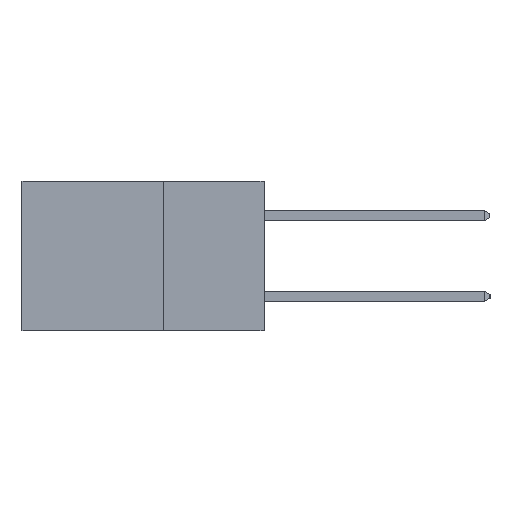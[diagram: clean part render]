
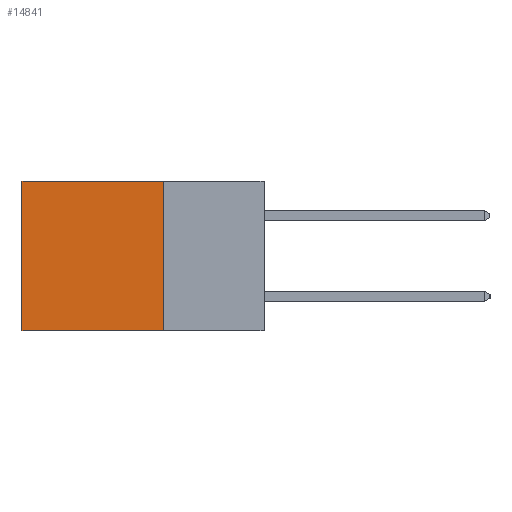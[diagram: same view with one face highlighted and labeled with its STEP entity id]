
A CAD part, left-side view. The second image highlights one B-rep face of the part: STEP entity #14841.
In plain terms, the highlighted planar face has unit normal (-1, 0, 0).
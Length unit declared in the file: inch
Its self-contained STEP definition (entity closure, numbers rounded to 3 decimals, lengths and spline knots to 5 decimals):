
#730 = CARTESIAN_POINT ( 'NONE',  ( 0.2615, 0.25, 0. ) ) ;
#1875 = EDGE_CURVE ( 'NONE', #12482, #14997, #13092, .T. ) ;
#2426 = ORIENTED_EDGE ( 'NONE', *, *, #13868, .F. ) ;
#3345 = CARTESIAN_POINT ( 'NONE',  ( 0.2615, 0.25, -0.37 ) ) ;
#3673 = CARTESIAN_POINT ( 'NONE',  ( 0.2615, 0.25, -0.37 ) ) ;
#3950 = VECTOR ( 'NONE', #18124, 39.37008 ) ;
#4193 = DIRECTION ( 'NONE',  ( 0., 1., 0. ) ) ;
#4370 = LINE ( 'NONE', #14473, #9425 ) ;
#4944 = DIRECTION ( 'NONE',  ( 0., 1., 0. ) ) ;
#6300 = ORIENTED_EDGE ( 'NONE', *, *, #1875, .T. ) ;
#6714 = FACE_OUTER_BOUND ( 'NONE', #17057, .T. ) ;
#7048 = CARTESIAN_POINT ( 'NONE',  ( 0.2615, 0.6, -0.37 ) ) ;
#7773 = DIRECTION ( 'NONE',  ( 0., 0., -1. ) ) ;
#8792 = DIRECTION ( 'NONE',  ( 0., 0., -1. ) ) ;
#9290 = EDGE_CURVE ( 'NONE', #10775, #14510, #17656, .T. ) ;
#9425 = VECTOR ( 'NONE', #4193, 39.37008 ) ;
#10200 = DIRECTION ( 'NONE',  ( 1., 0., 0. ) ) ;
#10775 = VERTEX_POINT ( 'NONE', #730 ) ;
#10986 = VECTOR ( 'NONE', #4944, 39.37008 ) ;
#11901 = ORIENTED_EDGE ( 'NONE', *, *, #9290, .F. ) ;
#12482 = VERTEX_POINT ( 'NONE', #17178 ) ;
#13092 = LINE ( 'NONE', #17963, #3950 ) ;
#13142 = ORIENTED_EDGE ( 'NONE', *, *, #15497, .T. ) ;
#13157 = VECTOR ( 'NONE', #8792, 39.37008 ) ;
#13868 = EDGE_CURVE ( 'NONE', #14510, #14997, #4370, .T. ) ;
#14473 = CARTESIAN_POINT ( 'NONE',  ( 0.2615, 0.25, -0.37 ) ) ;
#14510 = VERTEX_POINT ( 'NONE', #17624 ) ;
#14841 = ADVANCED_FACE ( 'NONE', ( #6714 ), #20428, .F. ) ;
#14997 = VERTEX_POINT ( 'NONE', #7048 ) ;
#15228 = CARTESIAN_POINT ( 'NONE',  ( 0.2615, 0.25, 0. ) ) ;
#15497 = EDGE_CURVE ( 'NONE', #10775, #12482, #20046, .T. ) ;
#17057 = EDGE_LOOP ( 'NONE', ( #6300, #2426, #11901, #13142 ) ) ;
#17178 = CARTESIAN_POINT ( 'NONE',  ( 0.2615, 0.6, 0. ) ) ;
#17624 = CARTESIAN_POINT ( 'NONE',  ( 0.2615, 0.25, -0.37 ) ) ;
#17656 = LINE ( 'NONE', #3673, #13157 ) ;
#17963 = CARTESIAN_POINT ( 'NONE',  ( 0.2615, 0.6, -0.37 ) ) ;
#18124 = DIRECTION ( 'NONE',  ( 0., 0., -1. ) ) ;
#20046 = LINE ( 'NONE', #15228, #10986 ) ;
#20428 = PLANE ( 'NONE',  #20464 ) ;
#20464 = AXIS2_PLACEMENT_3D ( 'NONE', #3345, #10200, #7773 ) ;
